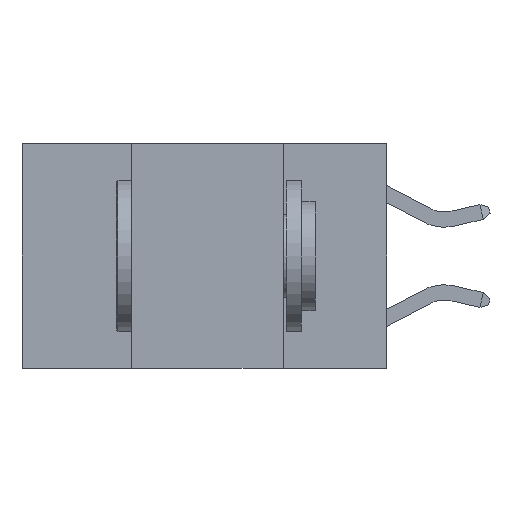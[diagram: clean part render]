
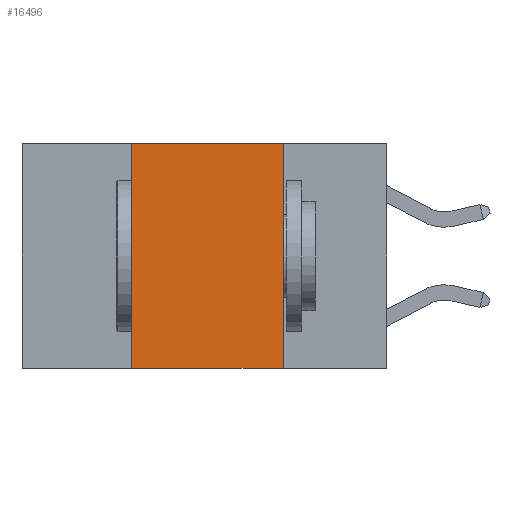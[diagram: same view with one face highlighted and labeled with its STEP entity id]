
A CAD part, left-side view. The second image highlights one B-rep face of the part: STEP entity #16496.
In plain terms, the highlighted planar face has unit normal (-1, 0, 0).
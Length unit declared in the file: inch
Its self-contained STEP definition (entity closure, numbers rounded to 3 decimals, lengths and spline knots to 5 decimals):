
#435 = LINE ( 'NONE', #17135, #15817 ) ;
#766 = ORIENTED_EDGE ( 'NONE', *, *, #24137, .T. ) ;
#1313 = EDGE_CURVE ( 'NONE', #19062, #14628, #435, .T. ) ;
#2057 = VECTOR ( 'NONE', #15952, 39.37008 ) ;
#2079 = LINE ( 'NONE', #23357, #18728 ) ;
#2731 = LINE ( 'NONE', #7596, #2057 ) ;
#3458 = CARTESIAN_POINT ( 'NONE',  ( 0., 0.17, 0. ) ) ;
#3629 = EDGE_CURVE ( 'NONE', #8668, #11173, #21576, .T. ) ;
#4613 = CARTESIAN_POINT ( 'NONE',  ( 0., 0.17, -0.37 ) ) ;
#4848 = CARTESIAN_POINT ( 'NONE',  ( 0., 0.6, 0. ) ) ;
#4975 = VECTOR ( 'NONE', #10740, 39.37008 ) ;
#5834 = CARTESIAN_POINT ( 'NONE',  ( 0., 0.42, -0.37 ) ) ;
#6338 = CARTESIAN_POINT ( 'NONE',  ( 0., 0.42, 0. ) ) ;
#7596 = CARTESIAN_POINT ( 'NONE',  ( 0., 0.6, 0. ) ) ;
#8267 = AXIS2_PLACEMENT_3D ( 'NONE', #4848, #25602, #13246 ) ;
#8377 = FACE_OUTER_BOUND ( 'NONE', #16194, .T. ) ;
#8668 = VERTEX_POINT ( 'NONE', #3458 ) ;
#8727 = CARTESIAN_POINT ( 'NONE',  ( 0., 0.17, 0. ) ) ;
#10740 = DIRECTION ( 'NONE',  ( 0., 0., -1. ) ) ;
#10934 = DIRECTION ( 'NONE',  ( 0., -1., 0. ) ) ;
#11173 = VERTEX_POINT ( 'NONE', #4613 ) ;
#13246 = DIRECTION ( 'NONE',  ( 0., 0., -1. ) ) ;
#14628 = VERTEX_POINT ( 'NONE', #6338 ) ;
#15817 = VECTOR ( 'NONE', #17260, 39.37008 ) ;
#15952 = DIRECTION ( 'NONE',  ( 0., -1., 0. ) ) ;
#16155 = ORIENTED_EDGE ( 'NONE', *, *, #20365, .F. ) ;
#16194 = EDGE_LOOP ( 'NONE', ( #21006, #16155, #16797, #766 ) ) ;
#16496 = ADVANCED_FACE ( 'NONE', ( #8377 ), #21486, .F. ) ;
#16797 = ORIENTED_EDGE ( 'NONE', *, *, #1313, .F. ) ;
#17135 = CARTESIAN_POINT ( 'NONE',  ( 0., 0.42, 0. ) ) ;
#17260 = DIRECTION ( 'NONE',  ( 0., 0., 1. ) ) ;
#18728 = VECTOR ( 'NONE', #10934, 39.37008 ) ;
#19062 = VERTEX_POINT ( 'NONE', #5834 ) ;
#20365 = EDGE_CURVE ( 'NONE', #14628, #8668, #2731, .T. ) ;
#21006 = ORIENTED_EDGE ( 'NONE', *, *, #3629, .F. ) ;
#21486 = PLANE ( 'NONE',  #8267 ) ;
#21576 = LINE ( 'NONE', #8727, #4975 ) ;
#23357 = CARTESIAN_POINT ( 'NONE',  ( 0., 0.6, -0.37 ) ) ;
#24137 = EDGE_CURVE ( 'NONE', #19062, #11173, #2079, .T. ) ;
#25602 = DIRECTION ( 'NONE',  ( 1., 0., 0. ) ) ;
